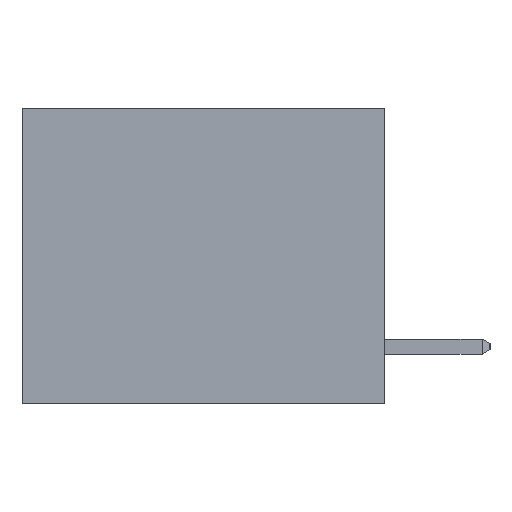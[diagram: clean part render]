
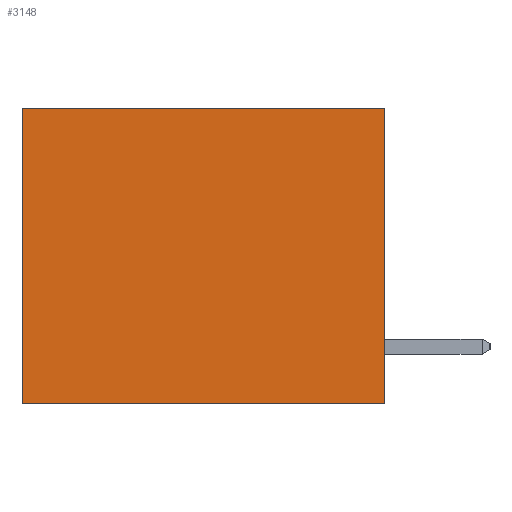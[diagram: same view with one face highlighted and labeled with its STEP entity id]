
A CAD part, left-side view. The second image highlights one B-rep face of the part: STEP entity #3148.
In plain terms, the highlighted planar face has unit normal (-1, 0, 0).
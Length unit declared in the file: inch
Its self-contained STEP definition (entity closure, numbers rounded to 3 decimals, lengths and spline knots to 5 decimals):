
#345 = EDGE_CURVE ( 'NONE', #5177, #13183, #9212, .T. ) ;
#379 = CARTESIAN_POINT ( 'NONE',  ( 0.3165, 0.6, 0. ) ) ;
#2136 = CARTESIAN_POINT ( 'NONE',  ( 0.3165, 0., -0.49 ) ) ;
#2414 = ORIENTED_EDGE ( 'NONE', *, *, #16157, .T. ) ;
#3148 = ADVANCED_FACE ( 'NONE', ( #13854 ), #9920, .F. ) ;
#5177 = VERTEX_POINT ( 'NONE', #13232 ) ;
#5679 = DIRECTION ( 'NONE',  ( 0., 0., -1. ) ) ;
#6938 = VECTOR ( 'NONE', #14571, 39.37008 ) ;
#7533 = LINE ( 'NONE', #8226, #6938 ) ;
#7607 = DIRECTION ( 'NONE',  ( 0., 1., 0. ) ) ;
#8154 = ORIENTED_EDGE ( 'NONE', *, *, #11110, .T. ) ;
#8226 = CARTESIAN_POINT ( 'NONE',  ( 0.3165, 0., 0. ) ) ;
#8733 = VERTEX_POINT ( 'NONE', #13907 ) ;
#8833 = VERTEX_POINT ( 'NONE', #379 ) ;
#9035 = CARTESIAN_POINT ( 'NONE',  ( 0.3165, 0.6, -0.49 ) ) ;
#9130 = LINE ( 'NONE', #11289, #10308 ) ;
#9212 = LINE ( 'NONE', #9394, #13740 ) ;
#9394 = CARTESIAN_POINT ( 'NONE',  ( 0.3165, 0., -0.49 ) ) ;
#9740 = DIRECTION ( 'NONE',  ( 0., 0., -1. ) ) ;
#9920 = PLANE ( 'NONE',  #13233 ) ;
#10308 = VECTOR ( 'NONE', #7607, 39.37008 ) ;
#10397 = DIRECTION ( 'NONE',  ( 0., 0., -1. ) ) ;
#10516 = LINE ( 'NONE', #9035, #15780 ) ;
#11110 = EDGE_CURVE ( 'NONE', #8833, #8733, #10516, .T. ) ;
#11289 = CARTESIAN_POINT ( 'NONE',  ( 0.3165, 0., -0.49 ) ) ;
#11541 = EDGE_LOOP ( 'NONE', ( #8154, #15563, #15192, #2414 ) ) ;
#11899 = CARTESIAN_POINT ( 'NONE',  ( 0.3165, 0., -0.49 ) ) ;
#12224 = DIRECTION ( 'NONE',  ( 1., 0., 0. ) ) ;
#13183 = VERTEX_POINT ( 'NONE', #11899 ) ;
#13232 = CARTESIAN_POINT ( 'NONE',  ( 0.3165, 0., 0. ) ) ;
#13233 = AXIS2_PLACEMENT_3D ( 'NONE', #2136, #12224, #9740 ) ;
#13740 = VECTOR ( 'NONE', #5679, 39.37008 ) ;
#13854 = FACE_OUTER_BOUND ( 'NONE', #11541, .T. ) ;
#13907 = CARTESIAN_POINT ( 'NONE',  ( 0.3165, 0.6, -0.49 ) ) ;
#14571 = DIRECTION ( 'NONE',  ( 0., 1., 0. ) ) ;
#15192 = ORIENTED_EDGE ( 'NONE', *, *, #345, .F. ) ;
#15563 = ORIENTED_EDGE ( 'NONE', *, *, #15674, .F. ) ;
#15674 = EDGE_CURVE ( 'NONE', #13183, #8733, #9130, .T. ) ;
#15780 = VECTOR ( 'NONE', #10397, 39.37008 ) ;
#16157 = EDGE_CURVE ( 'NONE', #5177, #8833, #7533, .T. ) ;
